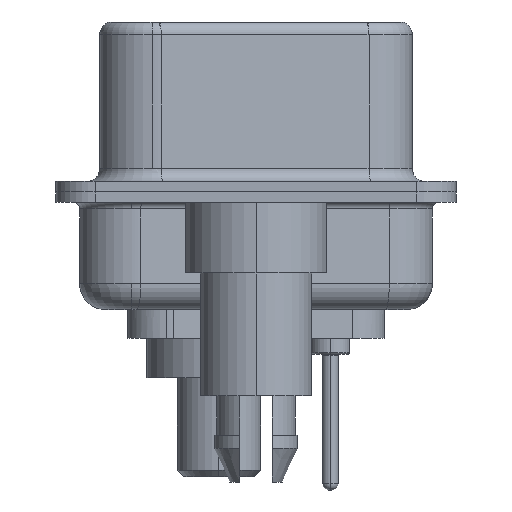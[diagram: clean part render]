
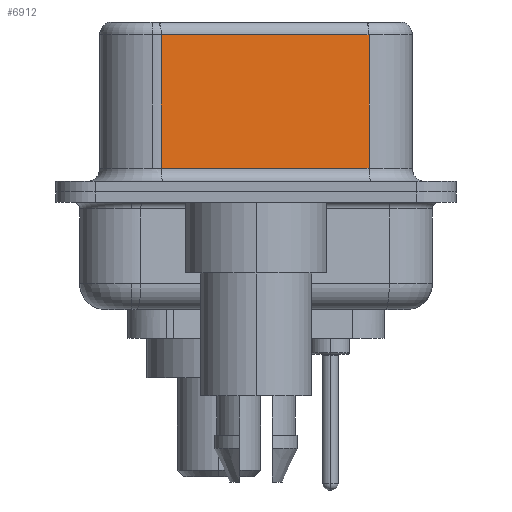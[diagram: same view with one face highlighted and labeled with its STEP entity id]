
A CAD part, left-side view. The second image highlights one B-rep face of the part: STEP entity #6912.
In plain terms, the highlighted planar face has unit normal (-0.985, -0.174, 0).
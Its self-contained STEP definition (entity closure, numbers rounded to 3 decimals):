
#262 = LINE ( 'NONE', #10538, #17339 ) ;
#544 = AXIS2_PLACEMENT_3D ( 'NONE', #4809, #15079, #4884 ) ;
#942 = FACE_OUTER_BOUND ( 'NONE', #20549, .T. ) ;
#1467 = VERTEX_POINT ( 'NONE', #19153 ) ;
#1651 = ORIENTED_EDGE ( 'NONE', *, *, #18023, .T. ) ;
#2069 = DIRECTION ( 'NONE',  ( -0.174, 0.985, 0. ) ) ;
#2423 = VECTOR ( 'NONE', #3904, 1000. ) ;
#2944 = ORIENTED_EDGE ( 'NONE', *, *, #13224, .T. ) ;
#3274 = EDGE_CURVE ( 'NONE', #17007, #5599, #14372, .T. ) ;
#3904 = DIRECTION ( 'NONE',  ( 0., 0., -1. ) ) ;
#3952 = EDGE_CURVE ( 'NONE', #1467, #8341, #16227, .T. ) ;
#4809 = CARTESIAN_POINT ( 'NONE',  ( 5.132, -4.322, 6.52 ) ) ;
#4884 = DIRECTION ( 'NONE',  ( -0.174, 0.985, 0. ) ) ;
#4893 = ORIENTED_EDGE ( 'NONE', *, *, #3274, .T. ) ;
#5599 = VERTEX_POINT ( 'NONE', #21272 ) ;
#6912 = ADVANCED_FACE ( 'NONE', ( #942 ), #13385, .F. ) ;
#7108 = VECTOR ( 'NONE', #20470, 1000. ) ;
#8341 = VERTEX_POINT ( 'NONE', #8899 ) ;
#8449 = CARTESIAN_POINT ( 'NONE',  ( 5.132, -4.322, 0.9 ) ) ;
#8899 = CARTESIAN_POINT ( 'NONE',  ( 5.132, -4.322, 0.9 ) ) ;
#9419 = CARTESIAN_POINT ( 'NONE',  ( 3.73, 3.628, 6.02 ) ) ;
#10538 = CARTESIAN_POINT ( 'NONE',  ( 5.132, -4.322, 6.02 ) ) ;
#11144 = VECTOR ( 'NONE', #15614, 1000. ) ;
#11617 = LINE ( 'NONE', #8449, #7108 ) ;
#13224 = EDGE_CURVE ( 'NONE', #5599, #8341, #11617, .T. ) ;
#13385 = PLANE ( 'NONE',  #544 ) ;
#14372 = LINE ( 'NONE', #16454, #2423 ) ;
#14742 = CARTESIAN_POINT ( 'NONE',  ( 5.132, -4.322, 6.52 ) ) ;
#15079 = DIRECTION ( 'NONE',  ( 0.985, 0.174, 0. ) ) ;
#15614 = DIRECTION ( 'NONE',  ( 0., 0., -1. ) ) ;
#16227 = LINE ( 'NONE', #14742, #11144 ) ;
#16454 = CARTESIAN_POINT ( 'NONE',  ( 3.73, 3.628, 6.52 ) ) ;
#17007 = VERTEX_POINT ( 'NONE', #9419 ) ;
#17339 = VECTOR ( 'NONE', #2069, 1000. ) ;
#18023 = EDGE_CURVE ( 'NONE', #1467, #17007, #262, .T. ) ;
#19153 = CARTESIAN_POINT ( 'NONE',  ( 5.132, -4.322, 6.02 ) ) ;
#20470 = DIRECTION ( 'NONE',  ( 0.174, -0.985, 0. ) ) ;
#20549 = EDGE_LOOP ( 'NONE', ( #21817, #1651, #4893, #2944 ) ) ;
#21272 = CARTESIAN_POINT ( 'NONE',  ( 3.73, 3.628, 0.9 ) ) ;
#21817 = ORIENTED_EDGE ( 'NONE', *, *, #3952, .F. ) ;
